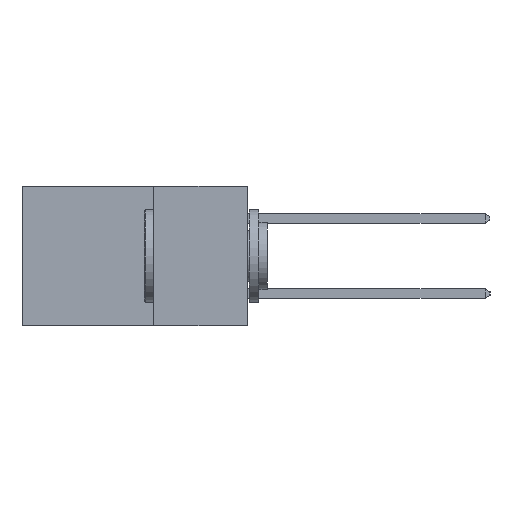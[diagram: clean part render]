
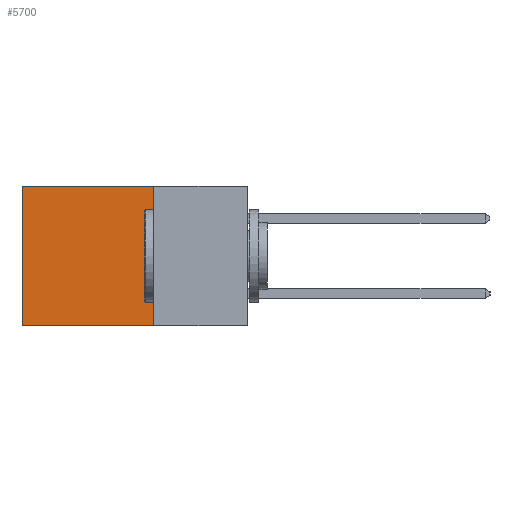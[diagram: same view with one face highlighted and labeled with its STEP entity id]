
A CAD part, left-side view. The second image highlights one B-rep face of the part: STEP entity #5700.
In plain terms, the highlighted planar face has unit normal (-1, 0, 0).
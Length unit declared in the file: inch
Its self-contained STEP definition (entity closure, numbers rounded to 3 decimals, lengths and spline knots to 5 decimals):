
#161 = CARTESIAN_POINT ( 'NONE',  ( 0.2615, 0.6, -0.37 ) ) ;
#935 = EDGE_CURVE ( 'NONE', #16996, #11232, #13219, .T. ) ;
#1720 = LINE ( 'NONE', #10706, #16826 ) ;
#1800 = DIRECTION ( 'NONE',  ( 0., 0., -1. ) ) ;
#2620 = VERTEX_POINT ( 'NONE', #5359 ) ;
#2759 = VECTOR ( 'NONE', #14327, 39.37008 ) ;
#3630 = FACE_OUTER_BOUND ( 'NONE', #7325, .T. ) ;
#3764 = VERTEX_POINT ( 'NONE', #16071 ) ;
#4125 = DIRECTION ( 'NONE',  ( 0., 0., -1. ) ) ;
#4242 = LINE ( 'NONE', #161, #7841 ) ;
#4398 = DIRECTION ( 'NONE',  ( 1., 0., 0. ) ) ;
#4419 = CARTESIAN_POINT ( 'NONE',  ( 0.2615, 0.25, -0.37 ) ) ;
#4479 = CARTESIAN_POINT ( 'NONE',  ( 0.2615, 0.25, -0.37 ) ) ;
#4604 = CARTESIAN_POINT ( 'NONE',  ( 0.2615, 0.25, 0. ) ) ;
#5359 = CARTESIAN_POINT ( 'NONE',  ( 0.2615, 0.6, 0. ) ) ;
#5672 = CARTESIAN_POINT ( 'NONE',  ( 0.2615, 0.25, 0. ) ) ;
#5700 = ADVANCED_FACE ( 'NONE', ( #3630 ), #11389, .F. ) ;
#7325 = EDGE_LOOP ( 'NONE', ( #15791, #8110, #12602, #13830 ) ) ;
#7841 = VECTOR ( 'NONE', #1800, 39.37008 ) ;
#8110 = ORIENTED_EDGE ( 'NONE', *, *, #17946, .F. ) ;
#9327 = DIRECTION ( 'NONE',  ( 0., 1., 0. ) ) ;
#9475 = VECTOR ( 'NONE', #13845, 39.37008 ) ;
#10706 = CARTESIAN_POINT ( 'NONE',  ( 0.2615, 0.25, -0.37 ) ) ;
#11232 = VERTEX_POINT ( 'NONE', #4479 ) ;
#11389 = PLANE ( 'NONE',  #15277 ) ;
#12602 = ORIENTED_EDGE ( 'NONE', *, *, #935, .F. ) ;
#13219 = LINE ( 'NONE', #13450, #9475 ) ;
#13450 = CARTESIAN_POINT ( 'NONE',  ( 0.2615, 0.25, -0.37 ) ) ;
#13562 = LINE ( 'NONE', #5672, #2759 ) ;
#13830 = ORIENTED_EDGE ( 'NONE', *, *, #16328, .T. ) ;
#13845 = DIRECTION ( 'NONE',  ( 0., 0., -1. ) ) ;
#14327 = DIRECTION ( 'NONE',  ( 0., 1., 0. ) ) ;
#14556 = EDGE_CURVE ( 'NONE', #2620, #3764, #4242, .T. ) ;
#15277 = AXIS2_PLACEMENT_3D ( 'NONE', #4419, #4398, #4125 ) ;
#15791 = ORIENTED_EDGE ( 'NONE', *, *, #14556, .T. ) ;
#16071 = CARTESIAN_POINT ( 'NONE',  ( 0.2615, 0.6, -0.37 ) ) ;
#16328 = EDGE_CURVE ( 'NONE', #16996, #2620, #13562, .T. ) ;
#16826 = VECTOR ( 'NONE', #9327, 39.37008 ) ;
#16996 = VERTEX_POINT ( 'NONE', #4604 ) ;
#17946 = EDGE_CURVE ( 'NONE', #11232, #3764, #1720, .T. ) ;
